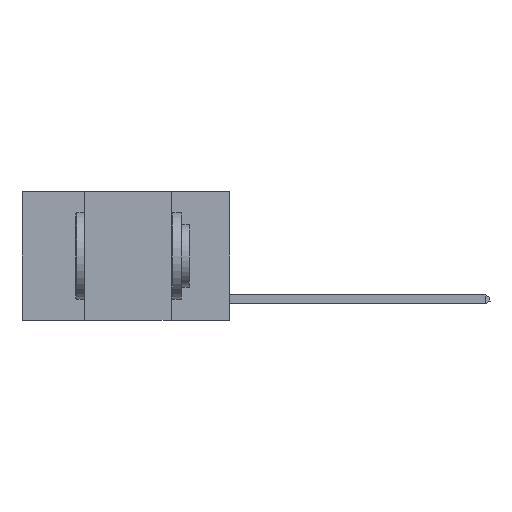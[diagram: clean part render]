
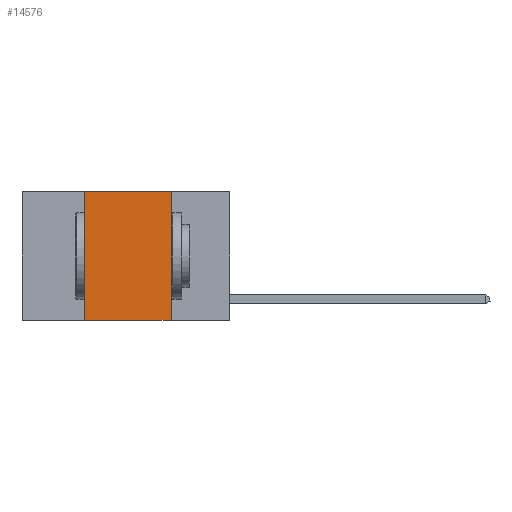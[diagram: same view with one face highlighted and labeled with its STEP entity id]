
A CAD part, left-side view. The second image highlights one B-rep face of the part: STEP entity #14576.
In plain terms, the highlighted planar face has unit normal (-1, 0, 0).
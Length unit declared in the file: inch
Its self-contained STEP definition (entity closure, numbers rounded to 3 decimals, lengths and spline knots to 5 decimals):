
#1158 = CARTESIAN_POINT ( 'NONE',  ( 0., 0.6, -0.37 ) ) ;
#1174 = VECTOR ( 'NONE', #5687, 39.37008 ) ;
#2182 = ORIENTED_EDGE ( 'NONE', *, *, #9413, .F. ) ;
#2814 = CARTESIAN_POINT ( 'NONE',  ( 0., 0.6, 0. ) ) ;
#2816 = LINE ( 'NONE', #1158, #3566 ) ;
#3566 = VECTOR ( 'NONE', #14693, 39.37008 ) ;
#3571 = LINE ( 'NONE', #14985, #7659 ) ;
#3636 = VERTEX_POINT ( 'NONE', #8804 ) ;
#3941 = CARTESIAN_POINT ( 'NONE',  ( 0., 0.6, 0. ) ) ;
#4014 = VERTEX_POINT ( 'NONE', #18998 ) ;
#5521 = EDGE_CURVE ( 'NONE', #3636, #13510, #12485, .T. ) ;
#5687 = DIRECTION ( 'NONE',  ( 0., 0., -1. ) ) ;
#5765 = EDGE_CURVE ( 'NONE', #12986, #3636, #14691, .T. ) ;
#6367 = AXIS2_PLACEMENT_3D ( 'NONE', #3941, #9147, #12714 ) ;
#7659 = VECTOR ( 'NONE', #15761, 39.37008 ) ;
#8483 = ORIENTED_EDGE ( 'NONE', *, *, #5765, .F. ) ;
#8804 = CARTESIAN_POINT ( 'NONE',  ( 0., 0.17, 0. ) ) ;
#9147 = DIRECTION ( 'NONE',  ( 1., 0., 0. ) ) ;
#9413 = EDGE_CURVE ( 'NONE', #4014, #12986, #3571, .T. ) ;
#11762 = ORIENTED_EDGE ( 'NONE', *, *, #14723, .T. ) ;
#12485 = LINE ( 'NONE', #21161, #1174 ) ;
#12714 = DIRECTION ( 'NONE',  ( 0., 0., -1. ) ) ;
#12986 = VERTEX_POINT ( 'NONE', #20274 ) ;
#13237 = VECTOR ( 'NONE', #16360, 39.37008 ) ;
#13510 = VERTEX_POINT ( 'NONE', #20545 ) ;
#14368 = FACE_OUTER_BOUND ( 'NONE', #19505, .T. ) ;
#14576 = ADVANCED_FACE ( 'NONE', ( #14368 ), #21163, .F. ) ;
#14691 = LINE ( 'NONE', #2814, #13237 ) ;
#14693 = DIRECTION ( 'NONE',  ( 0., -1., 0. ) ) ;
#14723 = EDGE_CURVE ( 'NONE', #4014, #13510, #2816, .T. ) ;
#14985 = CARTESIAN_POINT ( 'NONE',  ( 0., 0.42, 0. ) ) ;
#15761 = DIRECTION ( 'NONE',  ( 0., 0., 1. ) ) ;
#16360 = DIRECTION ( 'NONE',  ( 0., -1., 0. ) ) ;
#18431 = ORIENTED_EDGE ( 'NONE', *, *, #5521, .F. ) ;
#18998 = CARTESIAN_POINT ( 'NONE',  ( 0., 0.42, -0.37 ) ) ;
#19505 = EDGE_LOOP ( 'NONE', ( #18431, #8483, #2182, #11762 ) ) ;
#20274 = CARTESIAN_POINT ( 'NONE',  ( 0., 0.42, 0. ) ) ;
#20545 = CARTESIAN_POINT ( 'NONE',  ( 0., 0.17, -0.37 ) ) ;
#21161 = CARTESIAN_POINT ( 'NONE',  ( 0., 0.17, 0. ) ) ;
#21163 = PLANE ( 'NONE',  #6367 ) ;
